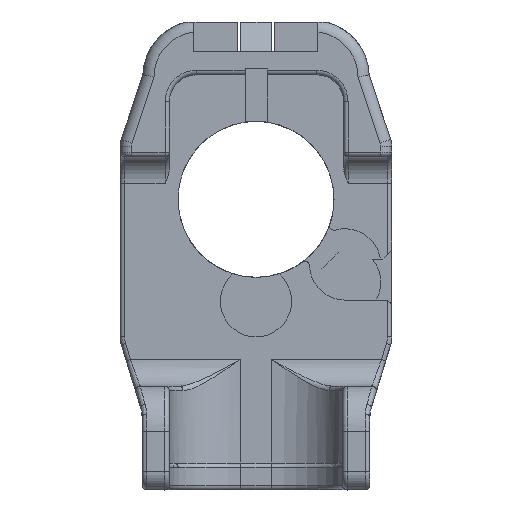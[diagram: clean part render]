
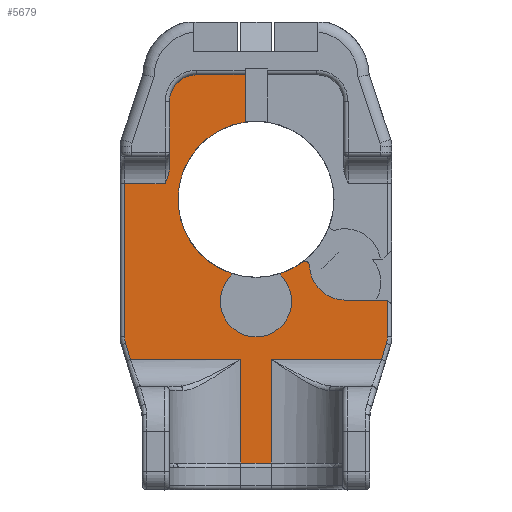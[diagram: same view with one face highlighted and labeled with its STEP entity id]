
A CAD part, front view. The second image highlights one B-rep face of the part: STEP entity #5679.
In plain terms, the highlighted planar face has unit normal (0, -1, 0).
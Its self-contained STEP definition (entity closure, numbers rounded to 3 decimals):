
#268=PLANE('',#6223);
#531=FACE_OUTER_BOUND('',#860,.T.);
#860=EDGE_LOOP('',(#4759,#4760,#4761,#4762,#4763,#4764,#4765,#4766,#4767,
#4768,#4769,#4770,#4771,#4772,#4773,#4774,#4775,#4776,#4777,#4778,#4779,
#4780,#4781));
#1059=CIRCLE('',#6033,2.5);
#1077=CIRCLE('',#6066,2.5);
#1139=CIRCLE('',#6189,4.);
#1152=CIRCLE('',#6206,4.);
#1153=CIRCLE('',#6213,0.5);
#1154=CIRCLE('',#6224,3.);
#1155=CIRCLE('',#6225,8.75);
#1156=CIRCLE('',#6226,8.75);
#1223=LINE('',#8337,#1679);
#1414=LINE('',#9618,#1870);
#1415=LINE('',#9631,#1871);
#1424=LINE('',#9709,#1880);
#1426=LINE('',#9721,#1882);
#1451=LINE('',#9856,#1907);
#1462=LINE('',#9950,#1918);
#1464=LINE('',#9960,#1920);
#1475=LINE('',#10049,#1931);
#1478=LINE('',#10053,#1934);
#1505=LINE('',#10215,#1961);
#1506=LINE('',#10219,#1962);
#1517=LINE('',#10261,#1973);
#1518=LINE('',#10267,#1974);
#1679=VECTOR('',#6472,10.);
#1870=VECTOR('',#7037,10.);
#1871=VECTOR('',#7052,10.);
#1880=VECTOR('',#7113,10.);
#1882=VECTOR('',#7127,10.);
#1907=VECTOR('',#7226,10.);
#1918=VECTOR('',#7281,10.);
#1920=VECTOR('',#7289,10.);
#1931=VECTOR('',#7348,10.);
#1934=VECTOR('',#7353,10.);
#1961=VECTOR('',#7486,10.);
#1962=VECTOR('',#7491,10.);
#1973=VECTOR('',#7526,10.);
#1974=VECTOR('',#7535,10.);
#2149=B_SPLINE_CURVE_WITH_KNOTS('',3,(#9688,#9689,#9690,#9691),
 .UNSPECIFIED.,.F.,.F.,(4,4),(0.382,0.56),
 .UNSPECIFIED.);
#2305=VERTEX_POINT('',#8334);
#2306=VERTEX_POINT('',#8336);
#2537=VERTEX_POINT('',#9615);
#2538=VERTEX_POINT('',#9617);
#2540=VERTEX_POINT('',#9622);
#2541=VERTEX_POINT('',#9624);
#2543=VERTEX_POINT('',#9630);
#2550=VERTEX_POINT('',#9687);
#2552=VERTEX_POINT('',#9707);
#2554=VERTEX_POINT('',#9713);
#2556=VERTEX_POINT('',#9719);
#2580=VERTEX_POINT('',#9846);
#2594=VERTEX_POINT('',#9940);
#2598=VERTEX_POINT('',#9957);
#2599=VERTEX_POINT('',#9959);
#2634=VERTEX_POINT('',#10166);
#2635=VERTEX_POINT('',#10168);
#2647=VERTEX_POINT('',#10201);
#2648=VERTEX_POINT('',#10203);
#2651=VERTEX_POINT('',#10213);
#2653=VERTEX_POINT('',#10224);
#2659=VERTEX_POINT('',#10259);
#2660=VERTEX_POINT('',#10263);
#2868=EDGE_CURVE('',#2305,#2306,#1223,.T.);
#3207=EDGE_CURVE('',#2537,#2538,#1414,.T.);
#3210=EDGE_CURVE('',#2540,#2541,#1059,.T.);
#3213=EDGE_CURVE('',#2541,#2543,#1415,.T.);
#3228=EDGE_CURVE('',#2538,#2550,#2149,.F.);
#3238=EDGE_CURVE('',#2552,#2537,#1424,.T.);
#3241=EDGE_CURVE('',#2554,#2552,#1077,.T.);
#3244=EDGE_CURVE('',#2556,#2554,#1426,.T.);
#3290=EDGE_CURVE('',#2556,#2580,#1451,.T.);
#3315=EDGE_CURVE('',#2594,#2543,#1462,.T.);
#3319=EDGE_CURVE('',#2599,#2598,#1464,.T.);
#3345=EDGE_CURVE('',#2599,#2580,#1475,.T.);
#3348=EDGE_CURVE('',#2594,#2598,#1478,.T.);
#3385=EDGE_CURVE('',#2635,#2634,#1139,.T.);
#3403=EDGE_CURVE('',#2648,#2647,#1152,.T.);
#3409=EDGE_CURVE('',#2648,#2651,#1505,.T.);
#3411=EDGE_CURVE('',#2651,#2540,#1506,.T.);
#3414=EDGE_CURVE('',#2653,#2647,#1153,.T.);
#3428=EDGE_CURVE('',#2659,#2550,#1517,.T.);
#3429=EDGE_CURVE('',#2660,#2659,#1154,.T.);
#3430=EDGE_CURVE('',#2653,#2635,#1155,.T.);
#3431=EDGE_CURVE('',#2634,#2306,#1156,.T.);
#3432=EDGE_CURVE('',#2305,#2660,#1518,.T.);
#4759=ORIENTED_EDGE('',*,*,#3429,.T.);
#4760=ORIENTED_EDGE('',*,*,#3428,.T.);
#4761=ORIENTED_EDGE('',*,*,#3228,.F.);
#4762=ORIENTED_EDGE('',*,*,#3207,.F.);
#4763=ORIENTED_EDGE('',*,*,#3238,.F.);
#4764=ORIENTED_EDGE('',*,*,#3241,.F.);
#4765=ORIENTED_EDGE('',*,*,#3244,.F.);
#4766=ORIENTED_EDGE('',*,*,#3290,.T.);
#4767=ORIENTED_EDGE('',*,*,#3345,.F.);
#4768=ORIENTED_EDGE('',*,*,#3319,.T.);
#4769=ORIENTED_EDGE('',*,*,#3348,.F.);
#4770=ORIENTED_EDGE('',*,*,#3315,.T.);
#4771=ORIENTED_EDGE('',*,*,#3213,.F.);
#4772=ORIENTED_EDGE('',*,*,#3210,.F.);
#4773=ORIENTED_EDGE('',*,*,#3411,.F.);
#4774=ORIENTED_EDGE('',*,*,#3409,.F.);
#4775=ORIENTED_EDGE('',*,*,#3403,.T.);
#4776=ORIENTED_EDGE('',*,*,#3414,.F.);
#4777=ORIENTED_EDGE('',*,*,#3430,.T.);
#4778=ORIENTED_EDGE('',*,*,#3385,.T.);
#4779=ORIENTED_EDGE('',*,*,#3431,.T.);
#4780=ORIENTED_EDGE('',*,*,#2868,.F.);
#4781=ORIENTED_EDGE('',*,*,#3432,.T.);
#5679=ADVANCED_FACE('',(#531),#268,.T.);
#6033=AXIS2_PLACEMENT_3D('',#9625,#7044,#7045);
#6066=AXIS2_PLACEMENT_3D('',#9715,#7120,#7121);
#6189=AXIS2_PLACEMENT_3D('',#10169,#7436,#7437);
#6206=AXIS2_PLACEMENT_3D('',#10204,#7475,#7476);
#6213=AXIS2_PLACEMENT_3D('',#10225,#7498,#7499);
#6223=AXIS2_PLACEMENT_3D('',#10262,#7527,#7528);
#6224=AXIS2_PLACEMENT_3D('',#10264,#7529,#7530);
#6225=AXIS2_PLACEMENT_3D('',#10265,#7531,#7532);
#6226=AXIS2_PLACEMENT_3D('',#10266,#7533,#7534);
#6472=DIRECTION('',(0.,0.,-1.));
#7037=DIRECTION('',(1.,0.,0.));
#7044=DIRECTION('center_axis',(0.,1.,0.));
#7045=DIRECTION('ref_axis',(0.989,0.,-0.149));
#7052=DIRECTION('',(-0.294,0.,-0.956));
#7113=DIRECTION('',(0.,0.,1.));
#7120=DIRECTION('center_axis',(0.,1.,0.));
#7121=DIRECTION('ref_axis',(-0.989,0.,-0.149));
#7127=DIRECTION('',(-0.294,0.,0.956));
#7226=DIRECTION('',(1.,0.,0.));
#7281=DIRECTION('',(1.,0.,0.));
#7289=DIRECTION('',(1.,0.,0.));
#7348=DIRECTION('',(0.,0.,1.));
#7353=DIRECTION('',(0.,0.,-1.));
#7436=DIRECTION('center_axis',(0.,1.,0.));
#7437=DIRECTION('ref_axis',(1.,0.,0.));
#7475=DIRECTION('center_axis',(0.,1.,0.));
#7476=DIRECTION('ref_axis',(-0.751,0.,0.66));
#7486=DIRECTION('',(1.,0.,0.));
#7491=DIRECTION('',(0.,0.,-1.));
#7498=DIRECTION('center_axis',(0.,1.,0.));
#7499=DIRECTION('ref_axis',(0.437,0.,0.9));
#7526=DIRECTION('',(0.,0.,-1.));
#7527=DIRECTION('center_axis',(0.,-1.,0.));
#7528=DIRECTION('ref_axis',(0.,0.,-1.));
#7529=DIRECTION('center_axis',(0.,-1.,0.));
#7530=DIRECTION('ref_axis',(-1.,0.,0.));
#7531=DIRECTION('center_axis',(0.,1.,0.));
#7532=DIRECTION('ref_axis',(-1.,0.,0.));
#7533=DIRECTION('center_axis',(0.,1.,0.));
#7534=DIRECTION('ref_axis',(-1.,0.,0.));
#7535=DIRECTION('',(-1.,0.,0.));
#8334=CARTESIAN_POINT('',(-1.212,65.024,-199.606));
#8336=CARTESIAN_POINT('',(-1.212,65.024,-204.904));
#8337=CARTESIAN_POINT('',(-1.212,65.024,-211.281));
#9615=CARTESIAN_POINT('',(-14.74,65.024,-211.805));
#9617=CARTESIAN_POINT('',(-10.192,65.024,-211.805));
#9618=CARTESIAN_POINT('',(-13.97,65.024,-211.805));
#9622=CARTESIAN_POINT('',(14.74,65.024,-228.994));
#9624=CARTESIAN_POINT('',(14.629,65.024,-229.729));
#9625=CARTESIAN_POINT('Origin',(12.24,65.024,-228.994));
#9630=CARTESIAN_POINT('',(14.077,65.024,-231.525));
#9631=CARTESIAN_POINT('',(16.519,65.024,-223.587));
#9687=CARTESIAN_POINT('',(-9.692,65.024,-210.002));
#9688=CARTESIAN_POINT('Ctrl Pts',(-9.692,65.024,-210.002));
#9689=CARTESIAN_POINT('Ctrl Pts',(-9.692,65.024,-210.597));
#9690=CARTESIAN_POINT('Ctrl Pts',(-9.968,65.024,-211.255));
#9691=CARTESIAN_POINT('Ctrl Pts',(-10.192,65.024,-211.805));
#9707=CARTESIAN_POINT('',(-14.74,65.024,-228.994));
#9709=CARTESIAN_POINT('',(-14.74,65.024,-215.95));
#9713=CARTESIAN_POINT('',(-14.629,65.024,-229.729));
#9715=CARTESIAN_POINT('Origin',(-12.24,65.024,-228.994));
#9719=CARTESIAN_POINT('',(-14.077,65.024,-231.525));
#9721=CARTESIAN_POINT('',(-15.078,65.024,-228.272));
#9846=CARTESIAN_POINT('',(-1.723,65.024,-231.525));
#9856=CARTESIAN_POINT('',(-10.795,65.024,-231.525));
#9940=CARTESIAN_POINT('',(1.723,65.024,-231.525));
#9950=CARTESIAN_POINT('',(1.27,65.024,-231.525));
#9957=CARTESIAN_POINT('',(1.723,65.024,-243.145));
#9959=CARTESIAN_POINT('',(-1.723,65.024,-243.145));
#9960=CARTESIAN_POINT('',(-6.35,65.024,-243.145));
#10049=CARTESIAN_POINT('',(-1.723,65.024,-233.763));
#10053=CARTESIAN_POINT('',(1.723,65.024,-226.066));
#10166=CARTESIAN_POINT('',(-2.569,65.024,-221.934));
#10168=CARTESIAN_POINT('',(2.569,65.024,-221.934));
#10169=CARTESIAN_POINT('Origin',(0.,65.024,-225.));
#10201=CARTESIAN_POINT('',(6.002,65.024,-220.991));
#10203=CARTESIAN_POINT('',(9.906,65.024,-224.871));
#10204=CARTESIAN_POINT('Origin',(10.,65.024,-220.872));
#10213=CARTESIAN_POINT('',(14.74,65.024,-224.871));
#10215=CARTESIAN_POINT('',(9.953,65.024,-224.871));
#10219=CARTESIAN_POINT('',(14.74,65.024,-215.945));
#10224=CARTESIAN_POINT('',(5.205,65.024,-220.604));
#10225=CARTESIAN_POINT('Origin',(5.502,65.024,-221.006));
#10259=CARTESIAN_POINT('',(-9.692,65.024,-202.606));
#10261=CARTESIAN_POINT('',(-9.692,65.024,-213.093));
#10262=CARTESIAN_POINT('Origin',(-12.7,65.024,-217.382));
#10263=CARTESIAN_POINT('',(-6.692,65.024,-199.606));
#10264=CARTESIAN_POINT('Origin',(-6.692,65.024,-202.606));
#10265=CARTESIAN_POINT('Origin',(0.,65.024,-213.57));
#10266=CARTESIAN_POINT('Origin',(0.,65.024,-213.57));
#10267=CARTESIAN_POINT('',(-12.701,65.024,-199.606));
